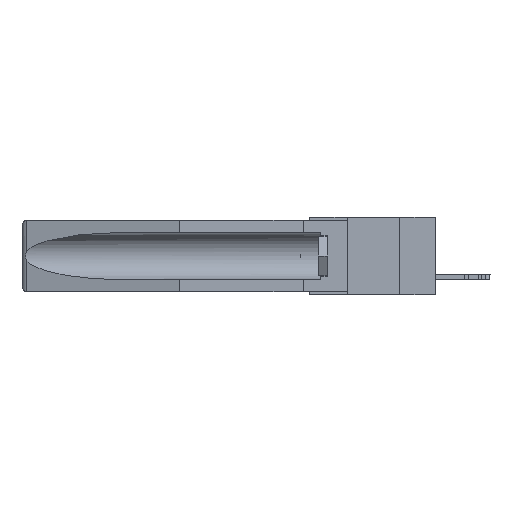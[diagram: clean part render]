
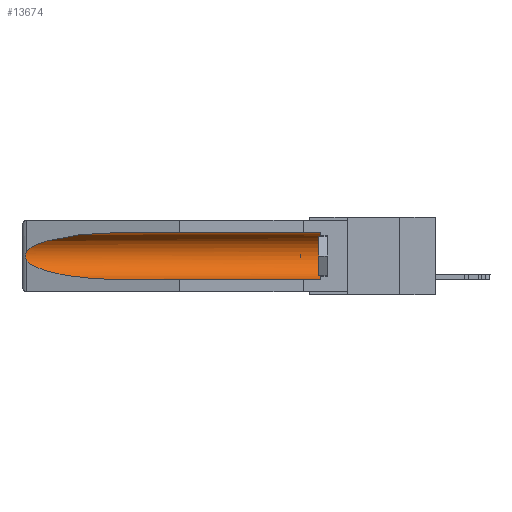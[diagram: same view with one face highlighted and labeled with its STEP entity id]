
A CAD part, left-side view. The second image highlights one B-rep face of the part: STEP entity #13674.
In plain terms, the highlighted cylindrical face has radius 2.857 mm (diameter 5.715 mm), a partial arc.
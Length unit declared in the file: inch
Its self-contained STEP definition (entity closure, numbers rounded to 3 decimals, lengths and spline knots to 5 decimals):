
#191 = CARTESIAN_POINT ( 'NONE',  ( 0.155, 1.07973, -0.059 ) ) ;
#507 = ORIENTED_EDGE ( 'NONE', *, *, #10907, .T. ) ;
#665 = CARTESIAN_POINT ( 'NONE',  ( 0.26537, 1.52718, -0.14972 ) ) ;
#1191 = CARTESIAN_POINT ( 'NONE',  ( 0.155, -0.30754, -0.284 ) ) ;
#1212 = CARTESIAN_POINT ( 'NONE',  ( 0.155, 0.126, -0.059 ) ) ;
#2620 = EDGE_LOOP ( 'NONE', ( #10787, #28333, #20038, #13950, #507, #10577 ) ) ;
#3247 = EDGE_CURVE ( 'NONE', #28204, #16770, #6117, .T. ) ;
#3765 = CARTESIAN_POINT ( 'NONE',  ( 0.26537, 1.52718, -0.19328 ) ) ;
#4481 = EDGE_CURVE ( 'NONE', #18496, #12229, #11070, .T. ) ;
#4627 = CYLINDRICAL_SURFACE ( 'NONE', #21286, 0.1125 ) ;
#4693 = CARTESIAN_POINT ( 'NONE',  ( 0.155, 0.126, -0.284 ) ) ;
#5206 = AXIS2_PLACEMENT_3D ( 'NONE', #32254, #27072, #11020 ) ;
#5442 = FACE_OUTER_BOUND ( 'NONE', #2620, .T. ) ;
#5648 = DIRECTION ( 'NONE',  ( 0., 1., 0. ) ) ;
#6117 = B_SPLINE_CURVE_WITH_KNOTS ( 'NONE', 3,
 ( #26316, #34282, #13153, #15249, #23503, #23278, #7610, #31630, #20617, #28998 ),
 .UNSPECIFIED., .F., .F.,
 ( 4, 2, 2, 2, 4 ),
 ( 0., 0.00029, 0.00058, 0.00087, 0.00117 ),
 .UNSPECIFIED. ) ;
#6547 =( BOUNDED_CURVE ( )  B_SPLINE_CURVE ( 3, ( #30772, #26538, #11373, #33813 ),
 .UNSPECIFIED., .F., .F. ) 
 B_SPLINE_CURVE_WITH_KNOTS ( ( 4, 4 ),
 ( 0.1948, 1.5708 ),
 .UNSPECIFIED. ) 
 CURVE ( )  GEOMETRIC_REPRESENTATION_ITEM ( )  RATIONAL_B_SPLINE_CURVE ( ( 1., 0.848, 0.848, 1. ) ) 
 REPRESENTATION_ITEM ( '' )  );
#7610 = CARTESIAN_POINT ( 'NONE',  ( 0.2673, 1.53269, -0.17917 ) ) ;
#8369 = DIRECTION ( 'NONE',  ( 0., 0., 1. ) ) ;
#9156 = LINE ( 'NONE', #1191, #10813 ) ;
#10577 = ORIENTED_EDGE ( 'NONE', *, *, #4481, .T. ) ;
#10787 = ORIENTED_EDGE ( 'NONE', *, *, #32814, .T. ) ;
#10813 = VECTOR ( 'NONE', #19507, 39.37008 ) ;
#10907 = EDGE_CURVE ( 'NONE', #30991, #18496, #13947, .T. ) ;
#11020 = DIRECTION ( 'NONE',  ( 0., 0., 1. ) ) ;
#11070 = LINE ( 'NONE', #19010, #22251 ) ;
#11373 = CARTESIAN_POINT ( 'NONE',  ( 0.21114, 1.30732, -0.284 ) ) ;
#11633 = CARTESIAN_POINT ( 'NONE',  ( 0.26537, 1.52718, -0.14972 ) ) ;
#12229 = VERTEX_POINT ( 'NONE', #28078 ) ;
#13153 = CARTESIAN_POINT ( 'NONE',  ( 0.26654, 1.53092, -0.15636 ) ) ;
#13674 = ADVANCED_FACE ( 'NONE', ( #5442 ), #4627, .F. ) ;
#13947 = CIRCLE ( 'NONE', #5206, 0.1125 ) ;
#13950 = ORIENTED_EDGE ( 'NONE', *, *, #14261, .F. ) ;
#14261 = EDGE_CURVE ( 'NONE', #30991, #22084, #9156, .T. ) ;
#15249 = CARTESIAN_POINT ( 'NONE',  ( 0.2673, 1.5327, -0.16383 ) ) ;
#16770 = VERTEX_POINT ( 'NONE', #3765 ) ;
#18496 = VERTEX_POINT ( 'NONE', #1212 ) ;
#18744 = CARTESIAN_POINT ( 'NONE',  ( 0.21114, 1.30732, -0.059 ) ) ;
#19010 = CARTESIAN_POINT ( 'NONE',  ( 0.155, -0.30754, -0.059 ) ) ;
#19507 = DIRECTION ( 'NONE',  ( 0., 1., 0. ) ) ;
#20038 = ORIENTED_EDGE ( 'NONE', *, *, #32709, .T. ) ;
#20617 = CARTESIAN_POINT ( 'NONE',  ( 0.26597, 1.5296, -0.19026 ) ) ;
#21023 =( BOUNDED_CURVE ( )  B_SPLINE_CURVE ( 3, ( #191, #18744, #27012, #665 ),
 .UNSPECIFIED., .F., .F. ) 
 B_SPLINE_CURVE_WITH_KNOTS ( ( 4, 4 ),
 ( 4.71239, 6.08839 ),
 .UNSPECIFIED. ) 
 CURVE ( )  GEOMETRIC_REPRESENTATION_ITEM ( )  RATIONAL_B_SPLINE_CURVE ( ( 1., 0.848, 0.848, 1. ) ) 
 REPRESENTATION_ITEM ( '' )  );
#21286 = AXIS2_PLACEMENT_3D ( 'NONE', #21703, #24496, #8369 ) ;
#21703 = CARTESIAN_POINT ( 'NONE',  ( 0.155, -0.30754, -0.1715 ) ) ;
#22084 = VERTEX_POINT ( 'NONE', #33459 ) ;
#22251 = VECTOR ( 'NONE', #5648, 39.37008 ) ;
#23278 = CARTESIAN_POINT ( 'NONE',  ( 0.2675, 1.53308, -0.17534 ) ) ;
#23503 = CARTESIAN_POINT ( 'NONE',  ( 0.2675, 1.53308, -0.16763 ) ) ;
#24496 = DIRECTION ( 'NONE',  ( 0., 1., 0. ) ) ;
#26316 = CARTESIAN_POINT ( 'NONE',  ( 0.26537, 1.52718, -0.14972 ) ) ;
#26538 = CARTESIAN_POINT ( 'NONE',  ( 0.25451, 1.48313, -0.24835 ) ) ;
#27012 = CARTESIAN_POINT ( 'NONE',  ( 0.25451, 1.48313, -0.09465 ) ) ;
#27072 = DIRECTION ( 'NONE',  ( 0., -1., 0. ) ) ;
#28078 = CARTESIAN_POINT ( 'NONE',  ( 0.155, 1.07973, -0.059 ) ) ;
#28204 = VERTEX_POINT ( 'NONE', #11633 ) ;
#28333 = ORIENTED_EDGE ( 'NONE', *, *, #3247, .T. ) ;
#28998 = CARTESIAN_POINT ( 'NONE',  ( 0.26537, 1.52718, -0.19328 ) ) ;
#30772 = CARTESIAN_POINT ( 'NONE',  ( 0.26537, 1.52718, -0.19328 ) ) ;
#30991 = VERTEX_POINT ( 'NONE', #4693 ) ;
#31630 = CARTESIAN_POINT ( 'NONE',  ( 0.26655, 1.53094, -0.18657 ) ) ;
#32254 = CARTESIAN_POINT ( 'NONE',  ( 0.155, 0.126, -0.1715 ) ) ;
#32709 = EDGE_CURVE ( 'NONE', #16770, #22084, #6547, .T. ) ;
#32814 = EDGE_CURVE ( 'NONE', #12229, #28204, #21023, .T. ) ;
#33459 = CARTESIAN_POINT ( 'NONE',  ( 0.155, 1.07973, -0.284 ) ) ;
#33813 = CARTESIAN_POINT ( 'NONE',  ( 0.155, 1.07973, -0.284 ) ) ;
#34282 = CARTESIAN_POINT ( 'NONE',  ( 0.26597, 1.52961, -0.15275 ) ) ;
